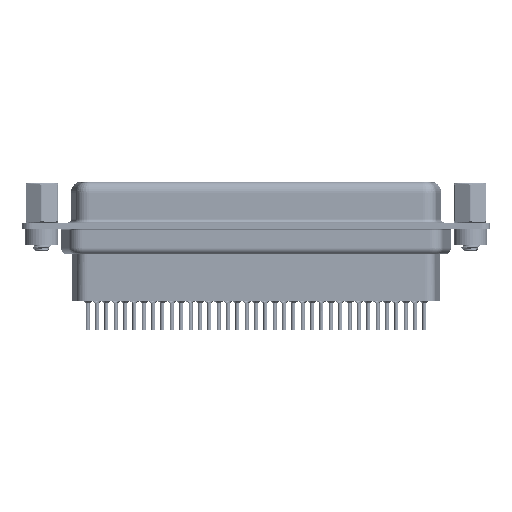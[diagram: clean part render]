
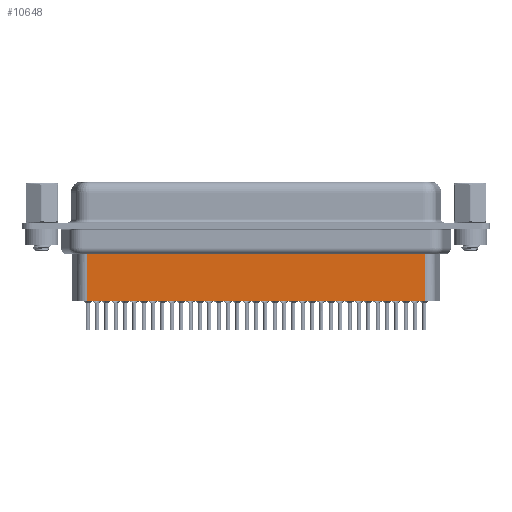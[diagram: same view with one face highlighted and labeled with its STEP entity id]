
A CAD part, front view. The second image highlights one B-rep face of the part: STEP entity #10648.
In plain terms, the highlighted planar face has unit normal (0, -1, 0).
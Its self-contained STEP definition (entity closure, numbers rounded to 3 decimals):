
#1256 = VECTOR ( 'NONE', #22411, 1000. ) ;
#2247 = LINE ( 'NONE', #16640, #22386 ) ;
#3031 = EDGE_CURVE ( 'NONE', #20876, #27872, #23895, .T. ) ;
#3725 = DIRECTION ( 'NONE',  ( 0., 0., -1. ) ) ;
#4451 = AXIS2_PLACEMENT_3D ( 'NONE', #24924, #22446, #19606 ) ;
#6191 = LINE ( 'NONE', #21326, #34280 ) ;
#7288 = EDGE_CURVE ( 'NONE', #27872, #23457, #23165, .T. ) ;
#8149 = VECTOR ( 'NONE', #32980, 1000. ) ;
#8201 = CARTESIAN_POINT ( 'NONE',  ( 6.706, -3.5, -3.1 ) ) ;
#9167 = CARTESIAN_POINT ( 'NONE',  ( 56.794, -3.5, -11.15 ) ) ;
#10648 = ADVANCED_FACE ( 'NONE', ( #19411 ), #16572, .T. ) ;
#12118 = ORIENTED_EDGE ( 'NONE', *, *, #3031, .T. ) ;
#14827 = EDGE_CURVE ( 'NONE', #20876, #36975, #6191, .T. ) ;
#15041 = CARTESIAN_POINT ( 'NONE',  ( 6.706, -3.5, -11.15 ) ) ;
#15582 = EDGE_LOOP ( 'NONE', ( #21968, #12118, #17475, #19682 ) ) ;
#16572 = PLANE ( 'NONE',  #4451 ) ;
#16640 = CARTESIAN_POINT ( 'NONE',  ( 6.706, -3.5, -11.15 ) ) ;
#17339 = CARTESIAN_POINT ( 'NONE',  ( 6.706, -3.5, -4.097 ) ) ;
#17475 = ORIENTED_EDGE ( 'NONE', *, *, #7288, .T. ) ;
#19411 = FACE_OUTER_BOUND ( 'NONE', #15582, .T. ) ;
#19606 = DIRECTION ( 'NONE',  ( 1., 0., 0. ) ) ;
#19682 = ORIENTED_EDGE ( 'NONE', *, *, #28576, .F. ) ;
#20876 = VERTEX_POINT ( 'NONE', #33809 ) ;
#21326 = CARTESIAN_POINT ( 'NONE',  ( 56.794, -3.5, -3.1 ) ) ;
#21968 = ORIENTED_EDGE ( 'NONE', *, *, #14827, .F. ) ;
#22386 = VECTOR ( 'NONE', #34473, 1000. ) ;
#22411 = DIRECTION ( 'NONE',  ( 0., 0., -1. ) ) ;
#22446 = DIRECTION ( 'NONE',  ( 0., -1., 0. ) ) ;
#23165 = LINE ( 'NONE', #8201, #1256 ) ;
#23457 = VERTEX_POINT ( 'NONE', #15041 ) ;
#23895 = LINE ( 'NONE', #35670, #8149 ) ;
#24924 = CARTESIAN_POINT ( 'NONE',  ( 6.706, -3.5, -3.1 ) ) ;
#27872 = VERTEX_POINT ( 'NONE', #17339 ) ;
#28576 = EDGE_CURVE ( 'NONE', #36975, #23457, #2247, .T. ) ;
#32980 = DIRECTION ( 'NONE',  ( -1., 0., 0. ) ) ;
#33809 = CARTESIAN_POINT ( 'NONE',  ( 56.794, -3.5, -4.097 ) ) ;
#34280 = VECTOR ( 'NONE', #3725, 1000. ) ;
#34473 = DIRECTION ( 'NONE',  ( -1., 0., 0. ) ) ;
#35670 = CARTESIAN_POINT ( 'NONE',  ( 6.459, -3.5, -4.097 ) ) ;
#36975 = VERTEX_POINT ( 'NONE', #9167 ) ;
